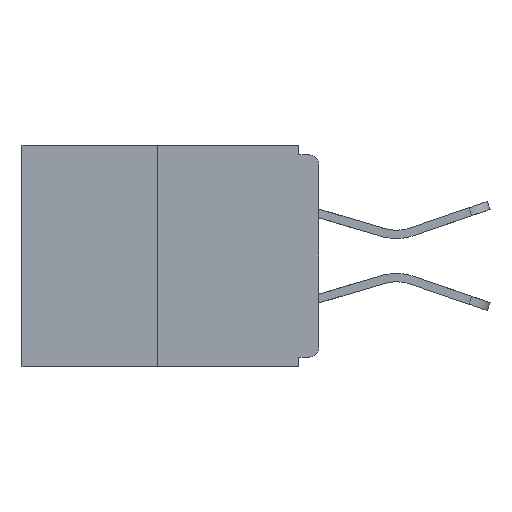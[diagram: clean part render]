
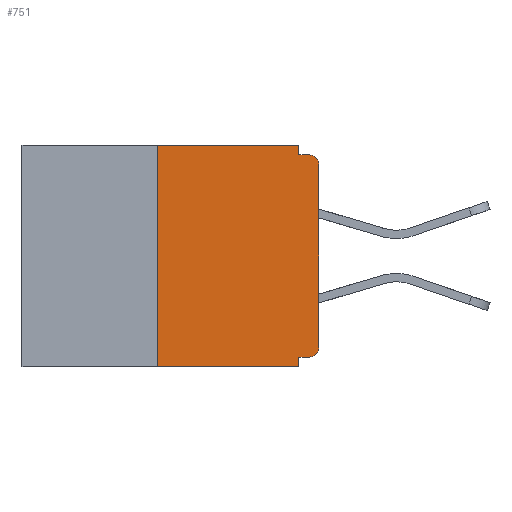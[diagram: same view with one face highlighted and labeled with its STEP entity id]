
A CAD part, left-side view. The second image highlights one B-rep face of the part: STEP entity #751.
In plain terms, the highlighted planar face has unit normal (-1, 0, 0).
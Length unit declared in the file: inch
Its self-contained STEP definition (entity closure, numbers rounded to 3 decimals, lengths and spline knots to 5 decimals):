
#737 = DIRECTION ( 'NONE',  ( 0., 0., 1. ) ) ;
#751 = ADVANCED_FACE ( 'NONE', ( #24839 ), #12209, .F. ) ;
#1171 = ORIENTED_EDGE ( 'NONE', *, *, #13112, .F. ) ;
#1360 = CIRCLE ( 'NONE', #4201, 0.015 ) ;
#1595 = VECTOR ( 'NONE', #22066, 39.37008 ) ;
#1877 = VECTOR ( 'NONE', #21326, 39.37008 ) ;
#2403 = VERTEX_POINT ( 'NONE', #9678 ) ;
#2529 = CARTESIAN_POINT ( 'NONE',  ( 0., 0.015, -0.03 ) ) ;
#2609 = VERTEX_POINT ( 'NONE', #17058 ) ;
#2774 = VECTOR ( 'NONE', #7812, 39.37008 ) ;
#2947 = CARTESIAN_POINT ( 'NONE',  ( 0., 0.015, -0.328 ) ) ;
#3066 = CARTESIAN_POINT ( 'NONE',  ( 0., 0.25, 0. ) ) ;
#3166 = VERTEX_POINT ( 'NONE', #17289 ) ;
#3169 = CARTESIAN_POINT ( 'NONE',  ( 0., 0., -0.015 ) ) ;
#4106 = AXIS2_PLACEMENT_3D ( 'NONE', #2529, #10848, #6784 ) ;
#4201 = AXIS2_PLACEMENT_3D ( 'NONE', #25513, #8285, #23030 ) ;
#4542 = EDGE_LOOP ( 'NONE', ( #19986, #9997, #16343, #27253, #19522, #24095, #21360, #6262, #10711, #1171 ) ) ;
#5200 = LINE ( 'NONE', #10371, #1877 ) ;
#5573 = CARTESIAN_POINT ( 'NONE',  ( 0., 0.031, -0.343 ) ) ;
#6262 = ORIENTED_EDGE ( 'NONE', *, *, #8090, .T. ) ;
#6416 = LINE ( 'NONE', #7343, #26544 ) ;
#6784 = DIRECTION ( 'NONE',  ( 0., 0., -1. ) ) ;
#6869 = CARTESIAN_POINT ( 'NONE',  ( 0., 0.46, -0.343 ) ) ;
#7343 = CARTESIAN_POINT ( 'NONE',  ( 0., 0.25, 0. ) ) ;
#7350 = CARTESIAN_POINT ( 'NONE',  ( 0., 0., 0. ) ) ;
#7812 = DIRECTION ( 'NONE',  ( 0., 0., 1. ) ) ;
#7958 = DIRECTION ( 'NONE',  ( 1., 0., 0. ) ) ;
#8090 = EDGE_CURVE ( 'NONE', #2609, #8146, #10498, .T. ) ;
#8146 = VERTEX_POINT ( 'NONE', #19777 ) ;
#8285 = DIRECTION ( 'NONE',  ( -1., 0., 0. ) ) ;
#8380 = EDGE_CURVE ( 'NONE', #22912, #19130, #5200, .T. ) ;
#8390 = LINE ( 'NONE', #20570, #15647 ) ;
#9678 = CARTESIAN_POINT ( 'NONE',  ( 0., 0.25, -0.343 ) ) ;
#9997 = ORIENTED_EDGE ( 'NONE', *, *, #16328, .F. ) ;
#10371 = CARTESIAN_POINT ( 'NONE',  ( 0., 0., -0.328 ) ) ;
#10498 = CIRCLE ( 'NONE', #4106, 0.015 ) ;
#10711 = ORIENTED_EDGE ( 'NONE', *, *, #11075, .F. ) ;
#10848 = DIRECTION ( 'NONE',  ( -1., 0., 0. ) ) ;
#11075 = EDGE_CURVE ( 'NONE', #16680, #8146, #14163, .T. ) ;
#11993 = CARTESIAN_POINT ( 'NONE',  ( 0., 0.031, -0.015 ) ) ;
#12209 = PLANE ( 'NONE',  #21987 ) ;
#13112 = EDGE_CURVE ( 'NONE', #17199, #16680, #19996, .T. ) ;
#13567 = VECTOR ( 'NONE', #21629, 39.37008 ) ;
#13966 = DIRECTION ( 'NONE',  ( 0., 0., -1. ) ) ;
#13988 = VERTEX_POINT ( 'NONE', #3066 ) ;
#14163 = LINE ( 'NONE', #3169, #1595 ) ;
#15378 = CARTESIAN_POINT ( 'NONE',  ( 0., 0., -0.313 ) ) ;
#15647 = VECTOR ( 'NONE', #18373, 39.37008 ) ;
#15733 = VECTOR ( 'NONE', #18344, 39.37008 ) ;
#15856 = EDGE_CURVE ( 'NONE', #2403, #3166, #18577, .T. ) ;
#16328 = EDGE_CURVE ( 'NONE', #2403, #13988, #6416, .T. ) ;
#16343 = ORIENTED_EDGE ( 'NONE', *, *, #15856, .T. ) ;
#16354 = CARTESIAN_POINT ( 'NONE',  ( 0., 0.46, 0. ) ) ;
#16599 = CARTESIAN_POINT ( 'NONE',  ( 0., 0.031, 0. ) ) ;
#16680 = VERTEX_POINT ( 'NONE', #11993 ) ;
#16819 = EDGE_CURVE ( 'NONE', #13988, #17199, #8390, .T. ) ;
#17058 = CARTESIAN_POINT ( 'NONE',  ( 0., 0., -0.03 ) ) ;
#17199 = VERTEX_POINT ( 'NONE', #23483 ) ;
#17289 = CARTESIAN_POINT ( 'NONE',  ( 0., 0.031, -0.343 ) ) ;
#18344 = DIRECTION ( 'NONE',  ( 0., 0., -1. ) ) ;
#18373 = DIRECTION ( 'NONE',  ( 0., -1., 0. ) ) ;
#18416 = EDGE_CURVE ( 'NONE', #22912, #22234, #1360, .T. ) ;
#18577 = LINE ( 'NONE', #6869, #13567 ) ;
#19060 = CARTESIAN_POINT ( 'NONE',  ( 0., 0.031, -0.328 ) ) ;
#19130 = VERTEX_POINT ( 'NONE', #19060 ) ;
#19522 = ORIENTED_EDGE ( 'NONE', *, *, #8380, .F. ) ;
#19777 = CARTESIAN_POINT ( 'NONE',  ( 0., 0.015, -0.015 ) ) ;
#19986 = ORIENTED_EDGE ( 'NONE', *, *, #16819, .F. ) ;
#19996 = LINE ( 'NONE', #16599, #15733 ) ;
#20227 = DIRECTION ( 'NONE',  ( 0., 0., -1. ) ) ;
#20570 = CARTESIAN_POINT ( 'NONE',  ( 0., 0.46, 0. ) ) ;
#21326 = DIRECTION ( 'NONE',  ( 0., 1., 0. ) ) ;
#21360 = ORIENTED_EDGE ( 'NONE', *, *, #26283, .T. ) ;
#21629 = DIRECTION ( 'NONE',  ( 0., -1., 0. ) ) ;
#21647 = VECTOR ( 'NONE', #20227, 39.37008 ) ;
#21987 = AXIS2_PLACEMENT_3D ( 'NONE', #16354, #7958, #13966 ) ;
#22066 = DIRECTION ( 'NONE',  ( 0., -1., 0. ) ) ;
#22234 = VERTEX_POINT ( 'NONE', #15378 ) ;
#22248 = LINE ( 'NONE', #7350, #2774 ) ;
#22912 = VERTEX_POINT ( 'NONE', #2947 ) ;
#23030 = DIRECTION ( 'NONE',  ( 0., 0., -1. ) ) ;
#23483 = CARTESIAN_POINT ( 'NONE',  ( 0., 0.031, 0. ) ) ;
#23640 = LINE ( 'NONE', #5573, #21647 ) ;
#24095 = ORIENTED_EDGE ( 'NONE', *, *, #18416, .T. ) ;
#24839 = FACE_OUTER_BOUND ( 'NONE', #4542, .T. ) ;
#25268 = EDGE_CURVE ( 'NONE', #19130, #3166, #23640, .T. ) ;
#25513 = CARTESIAN_POINT ( 'NONE',  ( 0., 0.015, -0.313 ) ) ;
#26283 = EDGE_CURVE ( 'NONE', #22234, #2609, #22248, .T. ) ;
#26544 = VECTOR ( 'NONE', #737, 39.37008 ) ;
#27253 = ORIENTED_EDGE ( 'NONE', *, *, #25268, .F. ) ;
